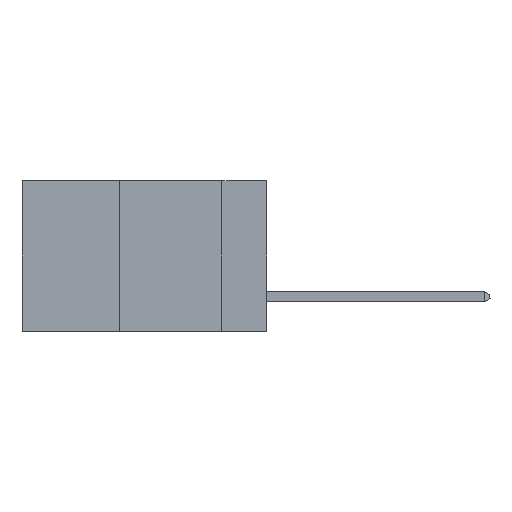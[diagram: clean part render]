
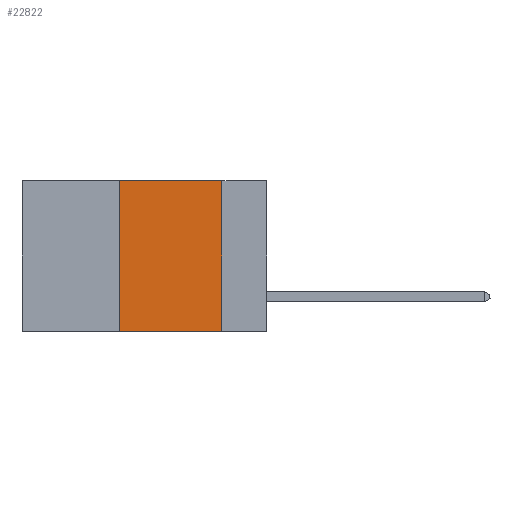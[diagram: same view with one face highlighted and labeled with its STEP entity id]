
A CAD part, left-side view. The second image highlights one B-rep face of the part: STEP entity #22822.
In plain terms, the highlighted planar face has unit normal (-1, 0, 0).
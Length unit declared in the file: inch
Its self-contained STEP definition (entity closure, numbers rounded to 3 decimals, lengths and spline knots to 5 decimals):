
#72 = DIRECTION ( 'NONE',  ( 0., 0., -1. ) ) ;
#187 = VERTEX_POINT ( 'NONE', #20589 ) ;
#657 = FACE_OUTER_BOUND ( 'NONE', #22654, .T. ) ;
#1564 = VECTOR ( 'NONE', #6523, 39.37008 ) ;
#1664 = EDGE_CURVE ( 'NONE', #7237, #187, #27028, .T. ) ;
#1669 = EDGE_CURVE ( 'NONE', #7847, #6199, #19086, .T. ) ;
#2316 = CARTESIAN_POINT ( 'NONE',  ( 0., 0.11, 0. ) ) ;
#2773 = ORIENTED_EDGE ( 'NONE', *, *, #1669, .F. ) ;
#3537 = VECTOR ( 'NONE', #26413, 39.37008 ) ;
#5233 = AXIS2_PLACEMENT_3D ( 'NONE', #20969, #21246, #72 ) ;
#5494 = LINE ( 'NONE', #20128, #3537 ) ;
#6199 = VERTEX_POINT ( 'NONE', #2316 ) ;
#6523 = DIRECTION ( 'NONE',  ( 0., -1., 0. ) ) ;
#7237 = VERTEX_POINT ( 'NONE', #9129 ) ;
#7507 = CARTESIAN_POINT ( 'NONE',  ( 0., 0.6, -0.37 ) ) ;
#7847 = VERTEX_POINT ( 'NONE', #18565 ) ;
#9129 = CARTESIAN_POINT ( 'NONE',  ( 0., 0.36, -0.37 ) ) ;
#11723 = ORIENTED_EDGE ( 'NONE', *, *, #1664, .T. ) ;
#13062 = EDGE_CURVE ( 'NONE', #6199, #187, #5494, .T. ) ;
#17189 = DIRECTION ( 'NONE',  ( 0., 0., 1. ) ) ;
#17617 = ORIENTED_EDGE ( 'NONE', *, *, #13062, .F. ) ;
#17761 = VECTOR ( 'NONE', #17189, 39.37008 ) ;
#18032 = CARTESIAN_POINT ( 'NONE',  ( 0., 0.6, 0. ) ) ;
#18433 = LINE ( 'NONE', #21574, #17761 ) ;
#18565 = CARTESIAN_POINT ( 'NONE',  ( 0., 0.36, 0. ) ) ;
#19081 = DIRECTION ( 'NONE',  ( 0., -1., 0. ) ) ;
#19086 = LINE ( 'NONE', #18032, #1564 ) ;
#19203 = PLANE ( 'NONE',  #5233 ) ;
#19378 = EDGE_CURVE ( 'NONE', #7237, #7847, #18433, .T. ) ;
#20128 = CARTESIAN_POINT ( 'NONE',  ( 0., 0.11, 0. ) ) ;
#20589 = CARTESIAN_POINT ( 'NONE',  ( 0., 0.11, -0.37 ) ) ;
#20969 = CARTESIAN_POINT ( 'NONE',  ( 0., 0.6, 0. ) ) ;
#21246 = DIRECTION ( 'NONE',  ( 1., 0., 0. ) ) ;
#21574 = CARTESIAN_POINT ( 'NONE',  ( 0., 0.36, 0. ) ) ;
#22654 = EDGE_LOOP ( 'NONE', ( #17617, #2773, #25125, #11723 ) ) ;
#22822 = ADVANCED_FACE ( 'NONE', ( #657 ), #19203, .F. ) ;
#25125 = ORIENTED_EDGE ( 'NONE', *, *, #19378, .F. ) ;
#25683 = VECTOR ( 'NONE', #19081, 39.37008 ) ;
#26413 = DIRECTION ( 'NONE',  ( 0., 0., -1. ) ) ;
#27028 = LINE ( 'NONE', #7507, #25683 ) ;
